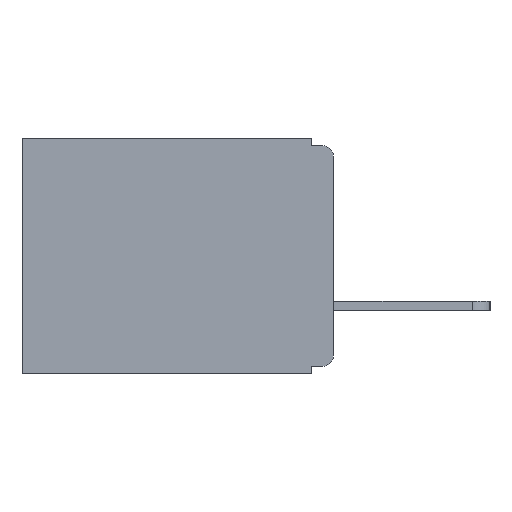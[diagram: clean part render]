
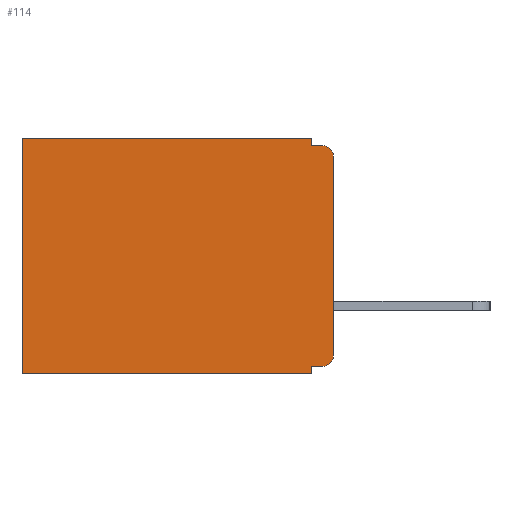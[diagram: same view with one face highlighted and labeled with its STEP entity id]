
A CAD part, left-side view. The second image highlights one B-rep face of the part: STEP entity #114.
In plain terms, the highlighted planar face has unit normal (-1, 0, 0).
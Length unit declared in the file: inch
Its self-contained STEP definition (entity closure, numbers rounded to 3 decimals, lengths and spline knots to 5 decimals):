
#114 = ADVANCED_FACE ( 'NONE', ( #3008 ), #22599, .F. ) ;
#409 = DIRECTION ( 'NONE',  ( 0., 0., -1. ) ) ;
#605 = DIRECTION ( 'NONE',  ( 0., 1., 0. ) ) ;
#1000 = VECTOR ( 'NONE', #18263, 39.37008 ) ;
#1151 = VERTEX_POINT ( 'NONE', #5029 ) ;
#1475 = ORIENTED_EDGE ( 'NONE', *, *, #18743, .F. ) ;
#2416 = VERTEX_POINT ( 'NONE', #17947 ) ;
#3008 = FACE_OUTER_BOUND ( 'NONE', #11202, .T. ) ;
#3122 = ORIENTED_EDGE ( 'NONE', *, *, #14048, .F. ) ;
#4612 = VECTOR ( 'NONE', #24372, 39.37008 ) ;
#4664 = VERTEX_POINT ( 'NONE', #12249 ) ;
#4829 = ORIENTED_EDGE ( 'NONE', *, *, #7722, .T. ) ;
#5029 = CARTESIAN_POINT ( 'NONE',  ( 0.3, 0.031, -0.32 ) ) ;
#5473 = EDGE_CURVE ( 'NONE', #11053, #24602, #17638, .T. ) ;
#6150 = CARTESIAN_POINT ( 'NONE',  ( 0.3, 0.015, -0.305 ) ) ;
#6205 = CARTESIAN_POINT ( 'NONE',  ( 0.3, 0.015, -0.01 ) ) ;
#6995 = LINE ( 'NONE', #24279, #1000 ) ;
#7083 = LINE ( 'NONE', #7635, #11282 ) ;
#7104 = VERTEX_POINT ( 'NONE', #10793 ) ;
#7635 = CARTESIAN_POINT ( 'NONE',  ( 0.3, 0., -0.33 ) ) ;
#7722 = EDGE_CURVE ( 'NONE', #12376, #9195, #24923, .T. ) ;
#7875 = ORIENTED_EDGE ( 'NONE', *, *, #5473, .T. ) ;
#8062 = ORIENTED_EDGE ( 'NONE', *, *, #22783, .F. ) ;
#8234 = DIRECTION ( 'NONE',  ( 0., 0., -1. ) ) ;
#8275 = CARTESIAN_POINT ( 'NONE',  ( 0.3, 0., -0.025 ) ) ;
#8326 = EDGE_CURVE ( 'NONE', #9195, #23877, #21108, .T. ) ;
#8664 = VERTEX_POINT ( 'NONE', #21729 ) ;
#9195 = VERTEX_POINT ( 'NONE', #17506 ) ;
#9974 = ORIENTED_EDGE ( 'NONE', *, *, #8326, .T. ) ;
#10397 = VECTOR ( 'NONE', #409, 39.37008 ) ;
#10446 = LINE ( 'NONE', #13527, #14627 ) ;
#10793 = CARTESIAN_POINT ( 'NONE',  ( 0.3, 0.031, -0.01 ) ) ;
#10975 = ORIENTED_EDGE ( 'NONE', *, *, #21528, .F. ) ;
#11053 = VERTEX_POINT ( 'NONE', #8275 ) ;
#11202 = EDGE_LOOP ( 'NONE', ( #1475, #7875, #3122, #25063, #4829, #9974, #8062, #11919, #10975, #13172 ) ) ;
#11282 = VECTOR ( 'NONE', #23803, 39.37008 ) ;
#11919 = ORIENTED_EDGE ( 'NONE', *, *, #20483, .F. ) ;
#12249 = CARTESIAN_POINT ( 'NONE',  ( 0.3, 0.015, -0.32 ) ) ;
#12289 = CARTESIAN_POINT ( 'NONE',  ( 0.3, 0., -0.33 ) ) ;
#12376 = VERTEX_POINT ( 'NONE', #14671 ) ;
#13172 = ORIENTED_EDGE ( 'NONE', *, *, #25844, .T. ) ;
#13527 = CARTESIAN_POINT ( 'NONE',  ( 0.3, 0.031, 0. ) ) ;
#13800 = CIRCLE ( 'NONE', #19738, 0.015 ) ;
#14048 = EDGE_CURVE ( 'NONE', #7104, #24602, #6995, .T. ) ;
#14122 = DIRECTION ( 'NONE',  ( -1., 0., 0. ) ) ;
#14299 = VECTOR ( 'NONE', #605, 39.37008 ) ;
#14376 = DIRECTION ( 'NONE',  ( 0., 1., 0. ) ) ;
#14627 = VECTOR ( 'NONE', #17549, 39.37008 ) ;
#14671 = CARTESIAN_POINT ( 'NONE',  ( 0.3, 0.031, 0. ) ) ;
#14895 = VECTOR ( 'NONE', #21622, 39.37008 ) ;
#15580 = AXIS2_PLACEMENT_3D ( 'NONE', #22619, #18889, #21976 ) ;
#16096 = VECTOR ( 'NONE', #14376, 39.37008 ) ;
#17506 = CARTESIAN_POINT ( 'NONE',  ( 0.3, 0.437, 0. ) ) ;
#17549 = DIRECTION ( 'NONE',  ( 0., 0., -1. ) ) ;
#17638 = CIRCLE ( 'NONE', #19980, 0.015 ) ;
#17947 = CARTESIAN_POINT ( 'NONE',  ( 0.3, 0.031, -0.33 ) ) ;
#18263 = DIRECTION ( 'NONE',  ( 0., -1., 0. ) ) ;
#18272 = CARTESIAN_POINT ( 'NONE',  ( 0.3, 0.015, -0.025 ) ) ;
#18743 = EDGE_CURVE ( 'NONE', #11053, #8664, #7083, .T. ) ;
#18889 = DIRECTION ( 'NONE',  ( 1., 0., 0. ) ) ;
#19738 = AXIS2_PLACEMENT_3D ( 'NONE', #6150, #20355, #8234 ) ;
#19824 = EDGE_CURVE ( 'NONE', #12376, #7104, #10446, .T. ) ;
#19980 = AXIS2_PLACEMENT_3D ( 'NONE', #18272, #14122, #24531 ) ;
#20265 = CARTESIAN_POINT ( 'NONE',  ( 0.3, 0.437, -0.33 ) ) ;
#20355 = DIRECTION ( 'NONE',  ( -1., 0., 0. ) ) ;
#20483 = EDGE_CURVE ( 'NONE', #1151, #2416, #25528, .T. ) ;
#20779 = LINE ( 'NONE', #22361, #4612 ) ;
#21108 = LINE ( 'NONE', #24646, #10397 ) ;
#21350 = LINE ( 'NONE', #12289, #16096 ) ;
#21528 = EDGE_CURVE ( 'NONE', #4664, #1151, #20779, .T. ) ;
#21622 = DIRECTION ( 'NONE',  ( 0., 0., -1. ) ) ;
#21729 = CARTESIAN_POINT ( 'NONE',  ( 0.3, 0., -0.305 ) ) ;
#21976 = DIRECTION ( 'NONE',  ( 0., 0., -1. ) ) ;
#22361 = CARTESIAN_POINT ( 'NONE',  ( 0.3, 0., -0.32 ) ) ;
#22599 = PLANE ( 'NONE',  #15580 ) ;
#22619 = CARTESIAN_POINT ( 'NONE',  ( 0.3, 0., -0.33 ) ) ;
#22783 = EDGE_CURVE ( 'NONE', #2416, #23877, #21350, .T. ) ;
#23630 = CARTESIAN_POINT ( 'NONE',  ( 0.3, 0.031, -0.33 ) ) ;
#23803 = DIRECTION ( 'NONE',  ( 0., 0., -1. ) ) ;
#23877 = VERTEX_POINT ( 'NONE', #20265 ) ;
#24279 = CARTESIAN_POINT ( 'NONE',  ( 0.3, 0., -0.01 ) ) ;
#24372 = DIRECTION ( 'NONE',  ( 0., 1., 0. ) ) ;
#24531 = DIRECTION ( 'NONE',  ( 0., 0., -1. ) ) ;
#24602 = VERTEX_POINT ( 'NONE', #6205 ) ;
#24646 = CARTESIAN_POINT ( 'NONE',  ( 0.3, 0.437, -0.33 ) ) ;
#24846 = CARTESIAN_POINT ( 'NONE',  ( 0.3, 0., 0. ) ) ;
#24923 = LINE ( 'NONE', #24846, #14299 ) ;
#25063 = ORIENTED_EDGE ( 'NONE', *, *, #19824, .F. ) ;
#25528 = LINE ( 'NONE', #23630, #14895 ) ;
#25844 = EDGE_CURVE ( 'NONE', #4664, #8664, #13800, .T. ) ;
